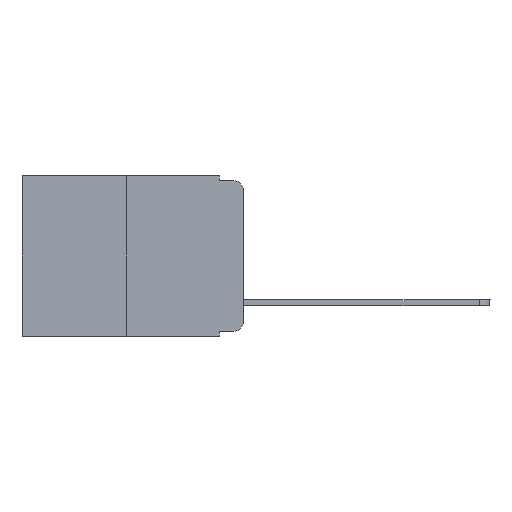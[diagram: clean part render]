
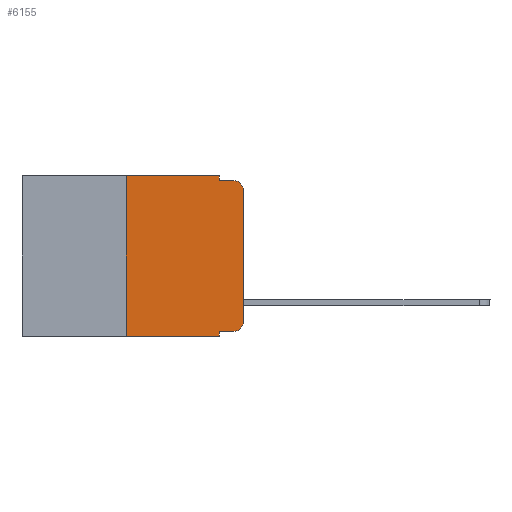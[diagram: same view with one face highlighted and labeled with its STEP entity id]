
A CAD part, left-side view. The second image highlights one B-rep face of the part: STEP entity #6155.
In plain terms, the highlighted planar face has unit normal (-1, 0, 0).
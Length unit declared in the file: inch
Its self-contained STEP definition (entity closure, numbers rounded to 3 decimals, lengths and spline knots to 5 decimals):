
#37 = CARTESIAN_POINT ( 'NONE',  ( 0., 0.02, -0.313 ) ) ;
#241 = ORIENTED_EDGE ( 'NONE', *, *, #8424, .T. ) ;
#352 = DIRECTION ( 'NONE',  ( 0., 0., 1. ) ) ;
#433 = CARTESIAN_POINT ( 'NONE',  ( 0., 0.25, 0. ) ) ;
#978 = ORIENTED_EDGE ( 'NONE', *, *, #19159, .T. ) ;
#1469 = LINE ( 'NONE', #19475, #9101 ) ;
#1678 = ORIENTED_EDGE ( 'NONE', *, *, #15209, .T. ) ;
#2126 = ORIENTED_EDGE ( 'NONE', *, *, #5731, .F. ) ;
#2163 = CIRCLE ( 'NONE', #20188, 0.02 ) ;
#2239 = EDGE_CURVE ( 'NONE', #3797, #11789, #14100, .T. ) ;
#2681 = ORIENTED_EDGE ( 'NONE', *, *, #20763, .F. ) ;
#3328 = VECTOR ( 'NONE', #3652, 39.37008 ) ;
#3584 = EDGE_CURVE ( 'NONE', #21947, #21593, #7846, .T. ) ;
#3596 = FACE_OUTER_BOUND ( 'NONE', #13413, .T. ) ;
#3652 = DIRECTION ( 'NONE',  ( 0., -1., 0. ) ) ;
#3797 = VERTEX_POINT ( 'NONE', #14645 ) ;
#4109 = CARTESIAN_POINT ( 'NONE',  ( 0., 0.051, -0.333 ) ) ;
#5123 = PLANE ( 'NONE',  #19529 ) ;
#5280 = VERTEX_POINT ( 'NONE', #12444 ) ;
#5731 = EDGE_CURVE ( 'NONE', #21947, #6945, #11780, .T. ) ;
#6120 = CARTESIAN_POINT ( 'NONE',  ( 0., 0.051, 0. ) ) ;
#6155 = ADVANCED_FACE ( 'NONE', ( #3596 ), #5123, .F. ) ;
#6289 = EDGE_CURVE ( 'NONE', #5280, #14213, #7983, .T. ) ;
#6585 = LINE ( 'NONE', #9630, #10714 ) ;
#6592 = CARTESIAN_POINT ( 'NONE',  ( 0., 0.02, -0.333 ) ) ;
#6945 = VERTEX_POINT ( 'NONE', #17425 ) ;
#6947 = CARTESIAN_POINT ( 'NONE',  ( 0., 0.051, -0.333 ) ) ;
#7717 = DIRECTION ( 'NONE',  ( 0., -1., 0. ) ) ;
#7846 = LINE ( 'NONE', #6947, #10528 ) ;
#7983 = LINE ( 'NONE', #12308, #3328 ) ;
#8424 = EDGE_CURVE ( 'NONE', #11789, #9673, #2163, .T. ) ;
#8490 = CARTESIAN_POINT ( 'NONE',  ( 0., 0.02, -0.03 ) ) ;
#8602 = DIRECTION ( 'NONE',  ( 0., 0., -1. ) ) ;
#8625 = ORIENTED_EDGE ( 'NONE', *, *, #6289, .F. ) ;
#8794 = CARTESIAN_POINT ( 'NONE',  ( 0., 0.473, -0.343 ) ) ;
#9101 = VECTOR ( 'NONE', #17827, 39.37008 ) ;
#9492 = CARTESIAN_POINT ( 'NONE',  ( 0., 0.25, -0.343 ) ) ;
#9630 = CARTESIAN_POINT ( 'NONE',  ( 0., 0.051, -0.01 ) ) ;
#9673 = VERTEX_POINT ( 'NONE', #10828 ) ;
#10528 = VECTOR ( 'NONE', #19113, 39.37008 ) ;
#10714 = VECTOR ( 'NONE', #7717, 39.37008 ) ;
#10755 = CIRCLE ( 'NONE', #12230, 0.02 ) ;
#10828 = CARTESIAN_POINT ( 'NONE',  ( 0., 0.02, -0.01 ) ) ;
#11150 = ORIENTED_EDGE ( 'NONE', *, *, #12477, .F. ) ;
#11344 = ORIENTED_EDGE ( 'NONE', *, *, #16335, .F. ) ;
#11448 = ORIENTED_EDGE ( 'NONE', *, *, #3584, .T. ) ;
#11612 = VERTEX_POINT ( 'NONE', #9492 ) ;
#11780 = LINE ( 'NONE', #6120, #19668 ) ;
#11789 = VERTEX_POINT ( 'NONE', #17773 ) ;
#12184 = VERTEX_POINT ( 'NONE', #15745 ) ;
#12187 = LINE ( 'NONE', #433, #17926 ) ;
#12230 = AXIS2_PLACEMENT_3D ( 'NONE', #37, #18851, #13694 ) ;
#12308 = CARTESIAN_POINT ( 'NONE',  ( 0., 0.473, 0. ) ) ;
#12444 = CARTESIAN_POINT ( 'NONE',  ( 0., 0.25, 0. ) ) ;
#12477 = EDGE_CURVE ( 'NONE', #12184, #9673, #6585, .T. ) ;
#12716 = ORIENTED_EDGE ( 'NONE', *, *, #2239, .T. ) ;
#13413 = EDGE_LOOP ( 'NONE', ( #12716, #241, #11150, #2681, #8625, #11344, #1678, #2126, #11448, #978 ) ) ;
#13694 = DIRECTION ( 'NONE',  ( 0., 0., -1. ) ) ;
#14070 = CARTESIAN_POINT ( 'NONE',  ( 0., 0.051, 0. ) ) ;
#14100 = LINE ( 'NONE', #18464, #20314 ) ;
#14213 = VERTEX_POINT ( 'NONE', #14070 ) ;
#14645 = CARTESIAN_POINT ( 'NONE',  ( 0., 0., -0.313 ) ) ;
#15024 = DIRECTION ( 'NONE',  ( 0., 0., 1. ) ) ;
#15209 = EDGE_CURVE ( 'NONE', #11612, #6945, #17724, .T. ) ;
#15294 = CARTESIAN_POINT ( 'NONE',  ( 0., 0.473, 0. ) ) ;
#15745 = CARTESIAN_POINT ( 'NONE',  ( 0., 0.051, -0.01 ) ) ;
#15783 = DIRECTION ( 'NONE',  ( 0., -1., 0. ) ) ;
#16335 = EDGE_CURVE ( 'NONE', #11612, #5280, #12187, .T. ) ;
#17425 = CARTESIAN_POINT ( 'NONE',  ( 0., 0.051, -0.343 ) ) ;
#17724 = LINE ( 'NONE', #8794, #20118 ) ;
#17773 = CARTESIAN_POINT ( 'NONE',  ( 0., 0., -0.03 ) ) ;
#17827 = DIRECTION ( 'NONE',  ( 0., 0., -1. ) ) ;
#17926 = VECTOR ( 'NONE', #352, 39.37008 ) ;
#18146 = DIRECTION ( 'NONE',  ( 0., 0., -1. ) ) ;
#18464 = CARTESIAN_POINT ( 'NONE',  ( 0., 0., 0. ) ) ;
#18725 = DIRECTION ( 'NONE',  ( 1., 0., 0. ) ) ;
#18851 = DIRECTION ( 'NONE',  ( -1., 0., 0. ) ) ;
#19113 = DIRECTION ( 'NONE',  ( 0., -1., 0. ) ) ;
#19159 = EDGE_CURVE ( 'NONE', #21593, #3797, #10755, .T. ) ;
#19475 = CARTESIAN_POINT ( 'NONE',  ( 0., 0.051, 0. ) ) ;
#19529 = AXIS2_PLACEMENT_3D ( 'NONE', #15294, #18725, #8602 ) ;
#19668 = VECTOR ( 'NONE', #18146, 39.37008 ) ;
#20118 = VECTOR ( 'NONE', #15783, 39.37008 ) ;
#20188 = AXIS2_PLACEMENT_3D ( 'NONE', #8490, #20608, #21693 ) ;
#20314 = VECTOR ( 'NONE', #15024, 39.37008 ) ;
#20608 = DIRECTION ( 'NONE',  ( -1., 0., 0. ) ) ;
#20763 = EDGE_CURVE ( 'NONE', #14213, #12184, #1469, .T. ) ;
#21593 = VERTEX_POINT ( 'NONE', #6592 ) ;
#21693 = DIRECTION ( 'NONE',  ( 0., 0., -1. ) ) ;
#21947 = VERTEX_POINT ( 'NONE', #4109 ) ;
